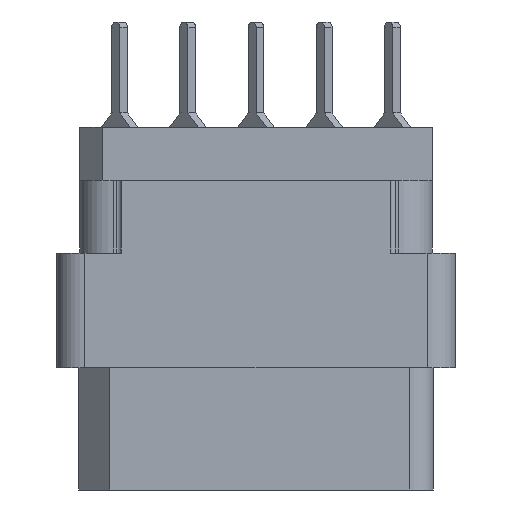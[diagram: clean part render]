
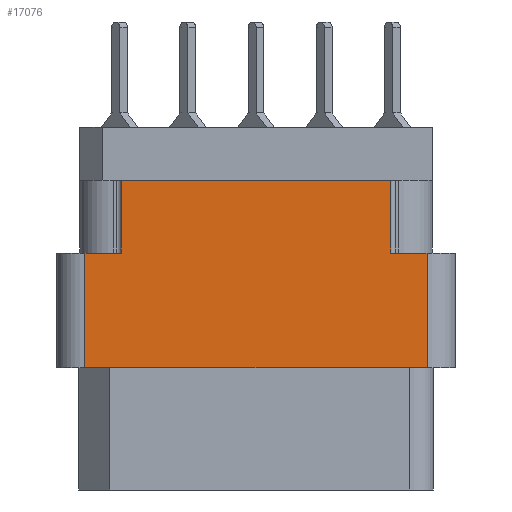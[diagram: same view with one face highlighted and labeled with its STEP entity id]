
A CAD part, left-side view. The second image highlights one B-rep face of the part: STEP entity #17076.
In plain terms, the highlighted planar face has unit normal (-1, 0, 0).
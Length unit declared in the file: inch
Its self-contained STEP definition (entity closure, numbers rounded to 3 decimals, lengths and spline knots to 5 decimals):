
#36 = LINE ( 'NONE', #8867, #11820 ) ;
#1463 = EDGE_CURVE ( 'NONE', #16304, #13947, #10999, .T. ) ;
#2721 = VECTOR ( 'NONE', #20620, 39.37008 ) ;
#2903 = VERTEX_POINT ( 'NONE', #26886 ) ;
#3731 = VERTEX_POINT ( 'NONE', #11017 ) ;
#3890 = CARTESIAN_POINT ( 'NONE',  ( -1., -0.376, -0.798 ) ) ;
#6650 = PLANE ( 'NONE',  #7982 ) ;
#7366 = DIRECTION ( 'NONE',  ( 0., 1., 0. ) ) ;
#7982 = AXIS2_PLACEMENT_3D ( 'NONE', #3890, #28719, #9589 ) ;
#8348 = ORIENTED_EDGE ( 'NONE', *, *, #17036, .F. ) ;
#8867 = CARTESIAN_POINT ( 'NONE',  ( -1., 0.438, -0.277 ) ) ;
#8915 = EDGE_CURVE ( 'NONE', #25883, #15254, #13772, .T. ) ;
#9589 = DIRECTION ( 'NONE',  ( 0., 0., 1. ) ) ;
#10146 = CARTESIAN_POINT ( 'NONE',  ( -1., 0.296, -0.277 ) ) ;
#10377 = VECTOR ( 'NONE', #30129, 39.37008 ) ;
#10484 = LINE ( 'NONE', #35301, #32082 ) ;
#10999 = LINE ( 'NONE', #10146, #32104 ) ;
#11017 = CARTESIAN_POINT ( 'NONE',  ( -1., -0.376, -0.277 ) ) ;
#11054 = ORIENTED_EDGE ( 'NONE', *, *, #14645, .F. ) ;
#11820 = VECTOR ( 'NONE', #22479, 39.37008 ) ;
#13275 = ORIENTED_EDGE ( 'NONE', *, *, #8915, .F. ) ;
#13772 = LINE ( 'NONE', #35829, #27915 ) ;
#13785 = VECTOR ( 'NONE', #30145, 39.37008 ) ;
#13947 = VERTEX_POINT ( 'NONE', #23421 ) ;
#14645 = EDGE_CURVE ( 'NONE', #2903, #3731, #27923, .T. ) ;
#14909 = LINE ( 'NONE', #23015, #2721 ) ;
#15254 = VERTEX_POINT ( 'NONE', #20662 ) ;
#15752 = VERTEX_POINT ( 'NONE', #28522 ) ;
#16208 = CARTESIAN_POINT ( 'NONE',  ( -1., -0.296, -0.277 ) ) ;
#16304 = VERTEX_POINT ( 'NONE', #34895 ) ;
#16502 = LINE ( 'NONE', #18900, #10377 ) ;
#16753 = LINE ( 'NONE', #16208, #22204 ) ;
#17036 = EDGE_CURVE ( 'NONE', #13947, #29713, #14909, .T. ) ;
#17076 = ADVANCED_FACE ( 'NONE', ( #23741 ), #6650, .T. ) ;
#17144 = EDGE_CURVE ( 'NONE', #15752, #25883, #10484, .T. ) ;
#18900 = CARTESIAN_POINT ( 'NONE',  ( -1., -0.376, -0.798 ) ) ;
#19000 = EDGE_CURVE ( 'NONE', #2903, #29713, #16753, .T. ) ;
#20620 = DIRECTION ( 'NONE',  ( 0., -1., 0. ) ) ;
#20662 = CARTESIAN_POINT ( 'NONE',  ( -1., 0.376, -0.277 ) ) ;
#21425 = EDGE_LOOP ( 'NONE', ( #13275, #33273, #27986, #11054, #35872, #8348, #32559, #35302 ) ) ;
#22204 = VECTOR ( 'NONE', #32938, 39.37008 ) ;
#22229 = CARTESIAN_POINT ( 'NONE',  ( -1., 0.376, -0.529 ) ) ;
#22479 = DIRECTION ( 'NONE',  ( 0., -1., 0. ) ) ;
#23015 = CARTESIAN_POINT ( 'NONE',  ( -1., 0.438, -0.117 ) ) ;
#23421 = CARTESIAN_POINT ( 'NONE',  ( -1., 0.296, -0.117 ) ) ;
#23741 = FACE_OUTER_BOUND ( 'NONE', #21425, .T. ) ;
#25368 = CARTESIAN_POINT ( 'NONE',  ( -1., -0.296, -0.277 ) ) ;
#25776 = EDGE_CURVE ( 'NONE', #15254, #16304, #36, .T. ) ;
#25883 = VERTEX_POINT ( 'NONE', #22229 ) ;
#25944 = CARTESIAN_POINT ( 'NONE',  ( -1., -0.296, -0.117 ) ) ;
#26886 = CARTESIAN_POINT ( 'NONE',  ( -1., -0.296, -0.277 ) ) ;
#27915 = VECTOR ( 'NONE', #36006, 39.37008 ) ;
#27923 = LINE ( 'NONE', #25368, #13785 ) ;
#27986 = ORIENTED_EDGE ( 'NONE', *, *, #33346, .T. ) ;
#28522 = CARTESIAN_POINT ( 'NONE',  ( -1., -0.376, -0.529 ) ) ;
#28719 = DIRECTION ( 'NONE',  ( -1., 0., 0. ) ) ;
#29713 = VERTEX_POINT ( 'NONE', #25944 ) ;
#30129 = DIRECTION ( 'NONE',  ( 0., 0., 1. ) ) ;
#30145 = DIRECTION ( 'NONE',  ( 0., -1., 0. ) ) ;
#30304 = DIRECTION ( 'NONE',  ( 0., 0., 1. ) ) ;
#32082 = VECTOR ( 'NONE', #7366, 39.37008 ) ;
#32104 = VECTOR ( 'NONE', #30304, 39.37008 ) ;
#32559 = ORIENTED_EDGE ( 'NONE', *, *, #1463, .F. ) ;
#32938 = DIRECTION ( 'NONE',  ( 0., 0., 1. ) ) ;
#33273 = ORIENTED_EDGE ( 'NONE', *, *, #17144, .F. ) ;
#33346 = EDGE_CURVE ( 'NONE', #15752, #3731, #16502, .T. ) ;
#34895 = CARTESIAN_POINT ( 'NONE',  ( -1., 0.296, -0.277 ) ) ;
#35301 = CARTESIAN_POINT ( 'NONE',  ( -1., -0.376, -0.529 ) ) ;
#35302 = ORIENTED_EDGE ( 'NONE', *, *, #25776, .F. ) ;
#35829 = CARTESIAN_POINT ( 'NONE',  ( -1., 0.376, -0.798 ) ) ;
#35872 = ORIENTED_EDGE ( 'NONE', *, *, #19000, .T. ) ;
#36006 = DIRECTION ( 'NONE',  ( 0., 0., 1. ) ) ;
